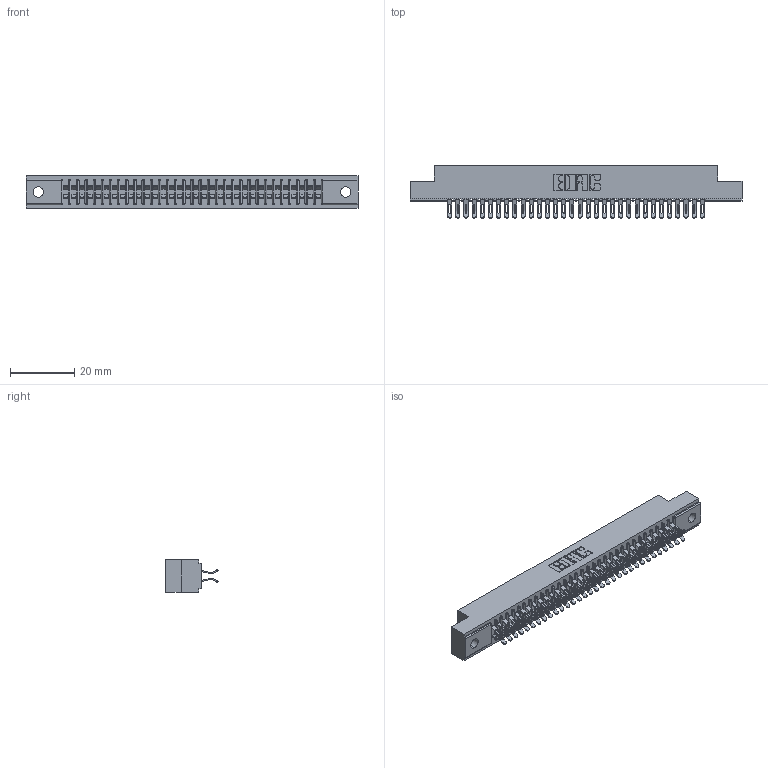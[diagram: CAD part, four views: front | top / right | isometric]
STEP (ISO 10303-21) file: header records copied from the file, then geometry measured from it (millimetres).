
FILE_DESCRIPTION (( 'STEP AP203' ), '1' );
FILE_NAME ('341-064-555-202.STEP', '2018-08-07T18:21:40', ( '' ), ( '' ), 'SwSTEP 2.0', 'SolidWorks 2016', '' );
FILE_SCHEMA (( 'CONFIG_CONTROL_DESIGN' ));
Length unit declared in the file: inch
Products named in the file (3): 341-292-001_341-292-155; 341-064-555-202; 341 Part_.128 (3.25) Dia Mounting Holes
Assembly tree (65 placements, depth 2):
  341-064-555-202
    341 Part_.128 (3.25) Dia Mounting Holes
    341-292-001_341-292-155  x64
Bounding box: 103.5 x 16.31 x 10.16 mm (x, y, z)
Volume: 7675.7 mm3; surface area: 13581.2 mm2
Topology: 65 solids, 65 shells, 5108 faces, 15260 edges, 9934 vertices
Faces by surface type: plane 2756, cylinder 2224, sphere 66, torus 62
Entity records: 40531 total; most frequent: CARTESIAN_POINT 6754, ORIENTED_EDGE 6700, DIRECTION 6552, EDGE_CURVE 3350, VECTOR 2680, LINE 2680, VERTEX_POINT 2122, AXIS2_PLACEMENT_3D 1936
